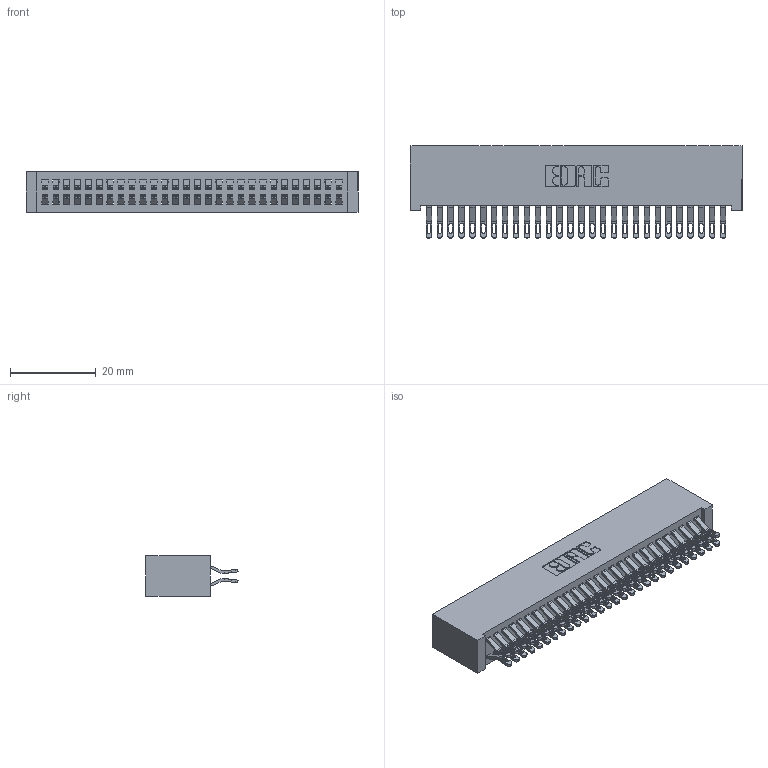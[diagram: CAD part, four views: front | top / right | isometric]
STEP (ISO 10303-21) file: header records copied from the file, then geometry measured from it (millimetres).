
FILE_DESCRIPTION (( 'STEP AP203' ), '1' );
FILE_NAME ('392-056-555-201.STEP', '2019-10-08T15:23:13', ( '' ), ( '' ), 'SwSTEP 2.0', 'SolidWorks 2016', '' );
FILE_SCHEMA (( 'CONFIG_CONTROL_DESIGN' ));
Length unit declared in the file: inch
Products named in the file (3): 392-056-555-201; 342 Part_Lugless; 345-292-001_555 Tail
Assembly tree (57 placements, depth 2):
  392-056-555-201
    342 Part_Lugless
    345-292-001_555 Tail  x56
Bounding box: 77.37 x 21.47 x 9.4 mm (x, y, z)
Volume: 7480.4 mm3; surface area: 12819.3 mm2
Topology: 57 solids, 57 shells, 3350 faces, 10523 edges, 7014 vertices
Faces by surface type: plane 1966, cylinder 1384
Entity records: 19741 total; most frequent: CARTESIAN_POINT 3320, ORIENTED_EDGE 3226, DIRECTION 2825, EDGE_CURVE 1613, LINE 1473, VECTOR 1473, VERTEX_POINT 1074, AXIS2_PLACEMENT_3D 676
